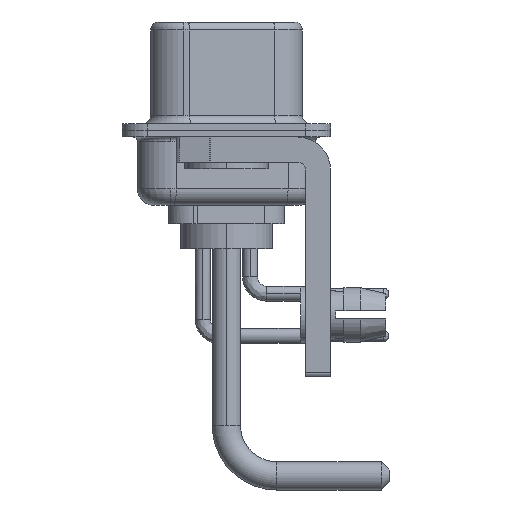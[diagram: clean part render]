
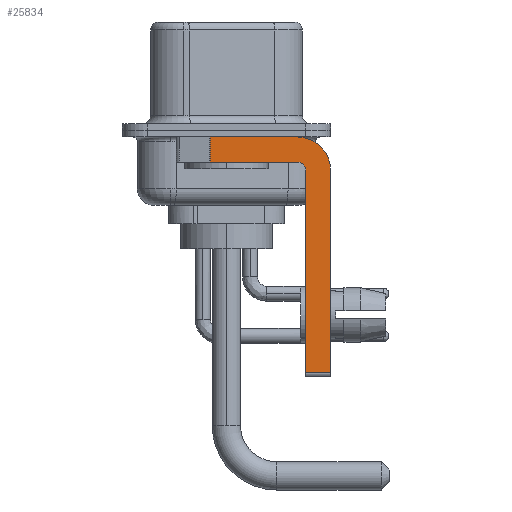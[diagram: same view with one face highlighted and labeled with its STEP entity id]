
A CAD part, left-side view. The second image highlights one B-rep face of the part: STEP entity #25834.
In plain terms, the highlighted planar face has unit normal (-1, 0, 0).
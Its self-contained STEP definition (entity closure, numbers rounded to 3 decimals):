
#491 = VERTEX_POINT ( 'NONE', #22445 ) ;
#506 = ORIENTED_EDGE ( 'NONE', *, *, #23423, .F. ) ;
#1999 = CARTESIAN_POINT ( 'NONE',  ( -2.9, -4.75, -14.55 ) ) ;
#2091 = EDGE_CURVE ( 'NONE', #17088, #12315, #24841, .T. ) ;
#2961 = DIRECTION ( 'NONE',  ( 0., 0., -1. ) ) ;
#3022 = VECTOR ( 'NONE', #13553, 1000. ) ;
#3174 = ORIENTED_EDGE ( 'NONE', *, *, #19513, .F. ) ;
#3349 = VECTOR ( 'NONE', #19960, 1000. ) ;
#3515 = FACE_OUTER_BOUND ( 'NONE', #19394, .T. ) ;
#3943 = ORIENTED_EDGE ( 'NONE', *, *, #22188, .T. ) ;
#4719 = VECTOR ( 'NONE', #21011, 1000. ) ;
#4864 = CIRCLE ( 'NONE', #14423, 2. ) ;
#5176 = CIRCLE ( 'NONE', #9102, 0.5 ) ;
#5735 = VERTEX_POINT ( 'NONE', #18127 ) ;
#5946 = DIRECTION ( 'NONE',  ( 1., 0., 0. ) ) ;
#6053 = VECTOR ( 'NONE', #9584, 1000. ) ;
#6235 = ORIENTED_EDGE ( 'NONE', *, *, #19003, .F. ) ;
#6291 = VERTEX_POINT ( 'NONE', #8748 ) ;
#6465 = CARTESIAN_POINT ( 'NONE',  ( -2.9, -6.25, -2.4 ) ) ;
#6593 = ORIENTED_EDGE ( 'NONE', *, *, #2091, .F. ) ;
#6671 = ORIENTED_EDGE ( 'NONE', *, *, #11484, .F. ) ;
#7765 = VERTEX_POINT ( 'NONE', #1999 ) ;
#8272 = PLANE ( 'NONE',  #20571 ) ;
#8494 = CARTESIAN_POINT ( 'NONE',  ( -2.9, 0.978, -1.9 ) ) ;
#8716 = DIRECTION ( 'NONE',  ( 1., 0., 0. ) ) ;
#8748 = CARTESIAN_POINT ( 'NONE',  ( -2.9, -6.25, -14.55 ) ) ;
#9102 = AXIS2_PLACEMENT_3D ( 'NONE', #19763, #13525, #15839 ) ;
#9243 = CARTESIAN_POINT ( 'NONE',  ( -2.9, -4.75, -14.8 ) ) ;
#9584 = DIRECTION ( 'NONE',  ( 0., -1., 0. ) ) ;
#9935 = CARTESIAN_POINT ( 'NONE',  ( -2.9, -4.25, -1.9 ) ) ;
#10066 = CARTESIAN_POINT ( 'NONE',  ( -2.9, -4.25, -1.9 ) ) ;
#11347 = VECTOR ( 'NONE', #26628, 1000. ) ;
#11484 = EDGE_CURVE ( 'NONE', #7765, #491, #19823, .T. ) ;
#12315 = VERTEX_POINT ( 'NONE', #8494 ) ;
#12478 = CARTESIAN_POINT ( 'NONE',  ( -2.9, 0.978, -0.4 ) ) ;
#12910 = CARTESIAN_POINT ( 'NONE',  ( -2.9, 3., -0.4 ) ) ;
#13094 = CARTESIAN_POINT ( 'NONE',  ( -2.9, -4.25, -0.4 ) ) ;
#13390 = LINE ( 'NONE', #19897, #6053 ) ;
#13525 = DIRECTION ( 'NONE',  ( -1., 0., 0. ) ) ;
#13553 = DIRECTION ( 'NONE',  ( 0., -1., 0. ) ) ;
#13645 = EDGE_CURVE ( 'NONE', #18775, #15866, #18999, .T. ) ;
#14423 = AXIS2_PLACEMENT_3D ( 'NONE', #16864, #8716, #21067 ) ;
#15839 = DIRECTION ( 'NONE',  ( 0., 0., 1. ) ) ;
#15866 = VERTEX_POINT ( 'NONE', #13094 ) ;
#16563 = DIRECTION ( 'NONE',  ( 0., 0., -1. ) ) ;
#16864 = CARTESIAN_POINT ( 'NONE',  ( -2.9, -4.25, -2.4 ) ) ;
#17088 = VERTEX_POINT ( 'NONE', #9935 ) ;
#17109 = CARTESIAN_POINT ( 'NONE',  ( -2.9, 0.978, -1.9 ) ) ;
#18127 = CARTESIAN_POINT ( 'NONE',  ( -2.9, -6.25, -2.4 ) ) ;
#18588 = CARTESIAN_POINT ( 'NONE',  ( -2.9, -4.25, -2.4 ) ) ;
#18775 = VERTEX_POINT ( 'NONE', #12478 ) ;
#18999 = LINE ( 'NONE', #12910, #3022 ) ;
#19003 = EDGE_CURVE ( 'NONE', #5735, #6291, #25084, .T. ) ;
#19394 = EDGE_LOOP ( 'NONE', ( #21154, #3943, #6593, #3174, #6671, #20855, #6235, #506 ) ) ;
#19513 = EDGE_CURVE ( 'NONE', #491, #17088, #5176, .T. ) ;
#19545 = VECTOR ( 'NONE', #2961, 1000. ) ;
#19580 = EDGE_CURVE ( 'NONE', #7765, #6291, #13390, .T. ) ;
#19763 = CARTESIAN_POINT ( 'NONE',  ( -2.9, -4.25, -2.4 ) ) ;
#19823 = LINE ( 'NONE', #9243, #3349 ) ;
#19897 = CARTESIAN_POINT ( 'NONE',  ( -2.9, -4.25, -14.55 ) ) ;
#19960 = DIRECTION ( 'NONE',  ( 0., 0., 1. ) ) ;
#20571 = AXIS2_PLACEMENT_3D ( 'NONE', #18588, #5946, #16563 ) ;
#20855 = ORIENTED_EDGE ( 'NONE', *, *, #19580, .T. ) ;
#21011 = DIRECTION ( 'NONE',  ( 0., 0., -1. ) ) ;
#21067 = DIRECTION ( 'NONE',  ( 0., 0., -1. ) ) ;
#21154 = ORIENTED_EDGE ( 'NONE', *, *, #13645, .F. ) ;
#21568 = LINE ( 'NONE', #17109, #19545 ) ;
#22188 = EDGE_CURVE ( 'NONE', #18775, #12315, #21568, .T. ) ;
#22445 = CARTESIAN_POINT ( 'NONE',  ( -2.9, -4.75, -2.4 ) ) ;
#23423 = EDGE_CURVE ( 'NONE', #15866, #5735, #4864, .T. ) ;
#24841 = LINE ( 'NONE', #10066, #11347 ) ;
#25084 = LINE ( 'NONE', #6465, #4719 ) ;
#25834 = ADVANCED_FACE ( 'NONE', ( #3515 ), #8272, .F. ) ;
#26628 = DIRECTION ( 'NONE',  ( 0., 1., 0. ) ) ;
